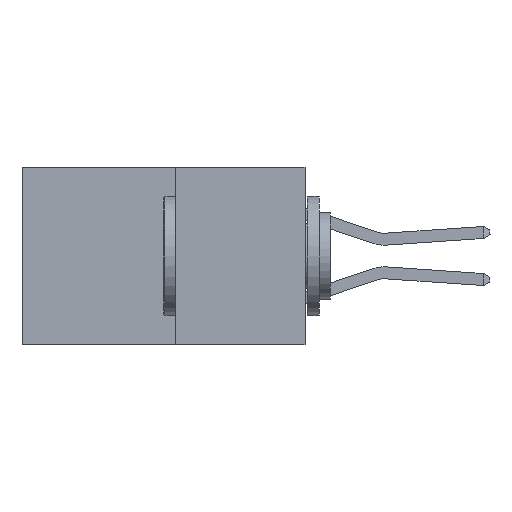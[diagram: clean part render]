
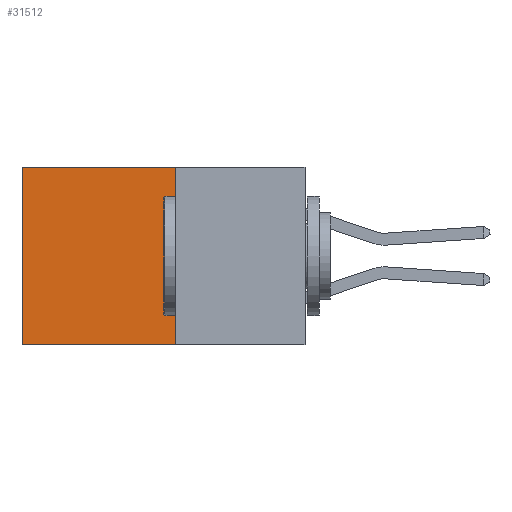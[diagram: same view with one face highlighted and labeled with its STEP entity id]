
A CAD part, left-side view. The second image highlights one B-rep face of the part: STEP entity #31512.
In plain terms, the highlighted planar face has unit normal (-1, 0, 0).
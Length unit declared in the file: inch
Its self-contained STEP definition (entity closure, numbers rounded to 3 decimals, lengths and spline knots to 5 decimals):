
#1010 = VERTEX_POINT ( 'NONE', #11303 ) ;
#1906 = CARTESIAN_POINT ( 'NONE',  ( 0.277, 0.59, 0. ) ) ;
#2819 = ORIENTED_EDGE ( 'NONE', *, *, #13534, .T. ) ;
#4328 = ORIENTED_EDGE ( 'NONE', *, *, #34340, .F. ) ;
#4523 = VERTEX_POINT ( 'NONE', #1906 ) ;
#5510 = EDGE_CURVE ( 'NONE', #14646, #1010, #12945, .T. ) ;
#5712 = VECTOR ( 'NONE', #23169, 39.37008 ) ;
#6271 = CARTESIAN_POINT ( 'NONE',  ( 0.277, 0.27, -0.37 ) ) ;
#7896 = VECTOR ( 'NONE', #10789, 39.37008 ) ;
#8552 = CARTESIAN_POINT ( 'NONE',  ( 0.277, 0.27, 0. ) ) ;
#8972 = DIRECTION ( 'NONE',  ( 1., 0., 0. ) ) ;
#10740 = FACE_OUTER_BOUND ( 'NONE', #29205, .T. ) ;
#10789 = DIRECTION ( 'NONE',  ( 0., 0., -1. ) ) ;
#11281 = DIRECTION ( 'NONE',  ( 0., 1., 0. ) ) ;
#11303 = CARTESIAN_POINT ( 'NONE',  ( 0.277, 0.59, -0.37 ) ) ;
#11555 = AXIS2_PLACEMENT_3D ( 'NONE', #6271, #8972, #27954 ) ;
#11648 = CARTESIAN_POINT ( 'NONE',  ( 0.277, 0.27, -0.37 ) ) ;
#11692 = ORIENTED_EDGE ( 'NONE', *, *, #30683, .T. ) ;
#12945 = LINE ( 'NONE', #23167, #5712 ) ;
#13534 = EDGE_CURVE ( 'NONE', #4523, #1010, #29512, .T. ) ;
#14646 = VERTEX_POINT ( 'NONE', #15758 ) ;
#15758 = CARTESIAN_POINT ( 'NONE',  ( 0.277, 0.27, -0.37 ) ) ;
#16088 = VECTOR ( 'NONE', #30671, 39.37008 ) ;
#21102 = VECTOR ( 'NONE', #11281, 39.37008 ) ;
#21294 = ORIENTED_EDGE ( 'NONE', *, *, #5510, .F. ) ;
#21953 = LINE ( 'NONE', #8552, #21102 ) ;
#22604 = PLANE ( 'NONE',  #11555 ) ;
#23167 = CARTESIAN_POINT ( 'NONE',  ( 0.277, 0.27, -0.37 ) ) ;
#23169 = DIRECTION ( 'NONE',  ( 0., 1., 0. ) ) ;
#23372 = LINE ( 'NONE', #11648, #16088 ) ;
#27954 = DIRECTION ( 'NONE',  ( 0., 0., -1. ) ) ;
#29205 = EDGE_LOOP ( 'NONE', ( #2819, #21294, #4328, #11692 ) ) ;
#29449 = CARTESIAN_POINT ( 'NONE',  ( 0.277, 0.27, 0. ) ) ;
#29512 = LINE ( 'NONE', #29737, #7896 ) ;
#29737 = CARTESIAN_POINT ( 'NONE',  ( 0.277, 0.59, -0.37 ) ) ;
#30671 = DIRECTION ( 'NONE',  ( 0., 0., -1. ) ) ;
#30683 = EDGE_CURVE ( 'NONE', #31938, #4523, #21953, .T. ) ;
#31512 = ADVANCED_FACE ( 'NONE', ( #10740 ), #22604, .F. ) ;
#31938 = VERTEX_POINT ( 'NONE', #29449 ) ;
#34340 = EDGE_CURVE ( 'NONE', #31938, #14646, #23372, .T. ) ;
